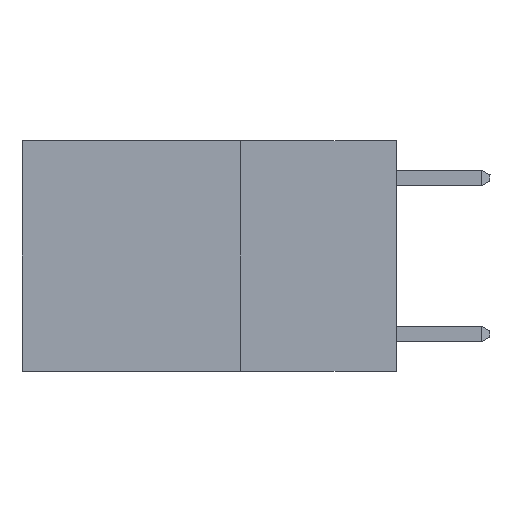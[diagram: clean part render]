
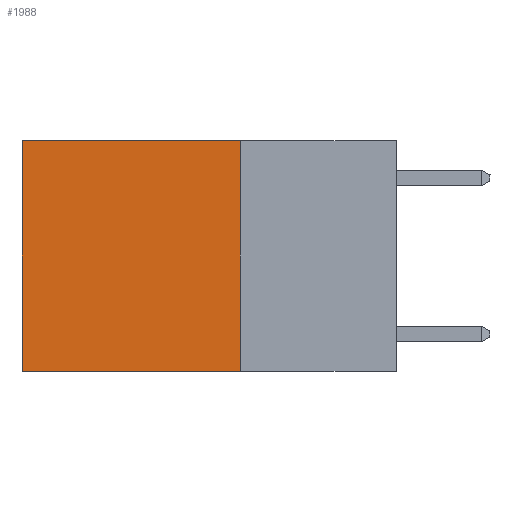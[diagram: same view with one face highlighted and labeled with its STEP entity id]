
A CAD part, left-side view. The second image highlights one B-rep face of the part: STEP entity #1988.
In plain terms, the highlighted planar face has unit normal (-1, 0, 0).
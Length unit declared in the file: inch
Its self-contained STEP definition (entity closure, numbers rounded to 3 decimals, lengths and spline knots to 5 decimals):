
#60 = EDGE_CURVE ( 'NONE', #6766, #3279, #2547, .T. ) ;
#214 = DIRECTION ( 'NONE',  ( 0., 0., -1. ) ) ;
#222 = ORIENTED_EDGE ( 'NONE', *, *, #1172, .T. ) ;
#389 = ORIENTED_EDGE ( 'NONE', *, *, #60, .T. ) ;
#547 = LINE ( 'NONE', #7403, #2850 ) ;
#731 = ORIENTED_EDGE ( 'NONE', *, *, #2212, .F. ) ;
#1124 = CARTESIAN_POINT ( 'NONE',  ( 0.2625, 0.6, 0. ) ) ;
#1172 = EDGE_CURVE ( 'NONE', #3167, #6766, #3130, .T. ) ;
#1359 = VECTOR ( 'NONE', #3972, 39.37008 ) ;
#1988 = ADVANCED_FACE ( 'NONE', ( #6679 ), #3259, .F. ) ;
#2212 = EDGE_CURVE ( 'NONE', #3167, #2952, #547, .T. ) ;
#2547 = LINE ( 'NONE', #1124, #1359 ) ;
#2615 = CARTESIAN_POINT ( 'NONE',  ( 0.2625, 0.25, -0.37 ) ) ;
#2624 = CARTESIAN_POINT ( 'NONE',  ( 0.2625, 0.25, 0. ) ) ;
#2666 = DIRECTION ( 'NONE',  ( 0., 1., 0. ) ) ;
#2850 = VECTOR ( 'NONE', #8541, 39.37008 ) ;
#2952 = VERTEX_POINT ( 'NONE', #9135 ) ;
#3130 = LINE ( 'NONE', #2624, #7857 ) ;
#3167 = VERTEX_POINT ( 'NONE', #4537 ) ;
#3259 = PLANE ( 'NONE',  #3890 ) ;
#3279 = VERTEX_POINT ( 'NONE', #8943 ) ;
#3334 = DIRECTION ( 'NONE',  ( 0., 1., 0. ) ) ;
#3832 = CARTESIAN_POINT ( 'NONE',  ( 0.2625, 0.25, 0. ) ) ;
#3890 = AXIS2_PLACEMENT_3D ( 'NONE', #3832, #7577, #214 ) ;
#3972 = DIRECTION ( 'NONE',  ( 0., 0., -1. ) ) ;
#4537 = CARTESIAN_POINT ( 'NONE',  ( 0.2625, 0.25, 0. ) ) ;
#4648 = CARTESIAN_POINT ( 'NONE',  ( 0.2625, 0.6, 0. ) ) ;
#5261 = EDGE_CURVE ( 'NONE', #2952, #3279, #6932, .T. ) ;
#6169 = VECTOR ( 'NONE', #2666, 39.37008 ) ;
#6679 = FACE_OUTER_BOUND ( 'NONE', #9093, .T. ) ;
#6766 = VERTEX_POINT ( 'NONE', #4648 ) ;
#6932 = LINE ( 'NONE', #2615, #6169 ) ;
#7403 = CARTESIAN_POINT ( 'NONE',  ( 0.2625, 0.25, 0. ) ) ;
#7575 = ORIENTED_EDGE ( 'NONE', *, *, #5261, .F. ) ;
#7577 = DIRECTION ( 'NONE',  ( 1., 0., 0. ) ) ;
#7857 = VECTOR ( 'NONE', #3334, 39.37008 ) ;
#8541 = DIRECTION ( 'NONE',  ( 0., 0., -1. ) ) ;
#8943 = CARTESIAN_POINT ( 'NONE',  ( 0.2625, 0.6, -0.37 ) ) ;
#9093 = EDGE_LOOP ( 'NONE', ( #389, #7575, #731, #222 ) ) ;
#9135 = CARTESIAN_POINT ( 'NONE',  ( 0.2625, 0.25, -0.37 ) ) ;
